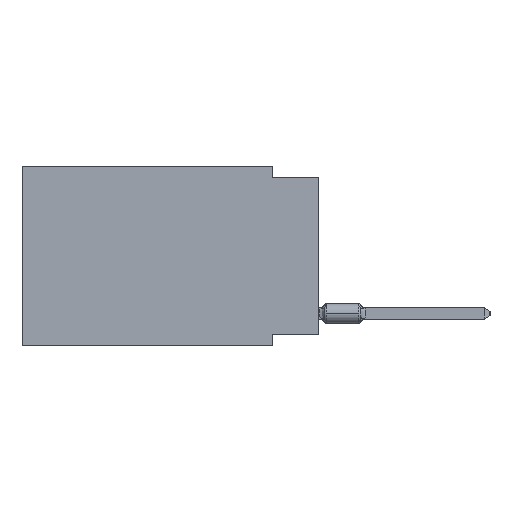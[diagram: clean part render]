
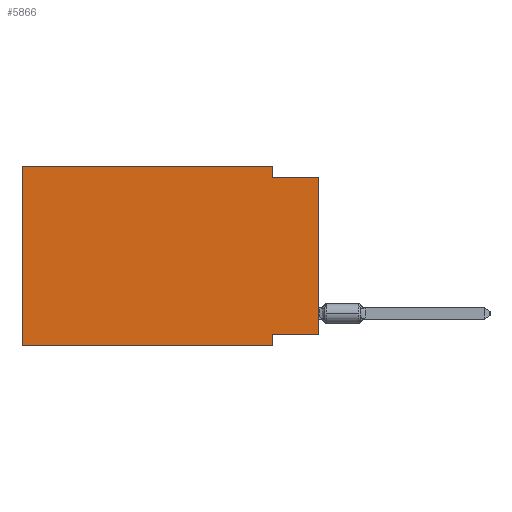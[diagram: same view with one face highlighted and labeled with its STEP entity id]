
A CAD part, left-side view. The second image highlights one B-rep face of the part: STEP entity #5866.
In plain terms, the highlighted planar face has unit normal (-1, 0, 0).
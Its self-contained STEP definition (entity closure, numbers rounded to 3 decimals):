
#885 = CARTESIAN_POINT ( 'NONE',  ( 0., 16.383, 0. ) ) ;
#1950 = CARTESIAN_POINT ( 'NONE',  ( 0., 0., -0.635 ) ) ;
#2306 = VECTOR ( 'NONE', #4783, 1000. ) ;
#2829 = EDGE_LOOP ( 'NONE', ( #25714, #37092, #14986, #3024, #22945, #7242, #21254, #27994 ) ) ;
#3024 = ORIENTED_EDGE ( 'NONE', *, *, #21896, .F. ) ;
#4580 = CARTESIAN_POINT ( 'NONE',  ( 0., 16.383, -9.906 ) ) ;
#4783 = DIRECTION ( 'NONE',  ( 0., -1., 0. ) ) ;
#4958 = DIRECTION ( 'NONE',  ( 0., 0., -1. ) ) ;
#5420 = DIRECTION ( 'NONE',  ( 0., 0., 1. ) ) ;
#5866 = ADVANCED_FACE ( 'NONE', ( #20929 ), #18463, .F. ) ;
#5921 = EDGE_CURVE ( 'NONE', #30603, #33404, #21854, .T. ) ;
#7242 = ORIENTED_EDGE ( 'NONE', *, *, #16509, .T. ) ;
#7796 = LINE ( 'NONE', #19370, #14177 ) ;
#8492 = CARTESIAN_POINT ( 'NONE',  ( 0., 2.54, -0.635 ) ) ;
#8503 = CARTESIAN_POINT ( 'NONE',  ( 0., 0., -9.271 ) ) ;
#9132 = DIRECTION ( 'NONE',  ( 0., 0., -1. ) ) ;
#9546 = CARTESIAN_POINT ( 'NONE',  ( 0., 0., -9.271 ) ) ;
#9736 = LINE ( 'NONE', #9546, #11423 ) ;
#10216 = VECTOR ( 'NONE', #9132, 1000. ) ;
#11132 = VERTEX_POINT ( 'NONE', #21292 ) ;
#11423 = VECTOR ( 'NONE', #21307, 1000. ) ;
#13697 = VECTOR ( 'NONE', #26478, 1000. ) ;
#14012 = CARTESIAN_POINT ( 'NONE',  ( 0., 0., -0.635 ) ) ;
#14177 = VECTOR ( 'NONE', #4958, 1000. ) ;
#14429 = CARTESIAN_POINT ( 'NONE',  ( 0., 2.54, -9.906 ) ) ;
#14469 = CARTESIAN_POINT ( 'NONE',  ( 0., 2.54, -9.271 ) ) ;
#14500 = EDGE_CURVE ( 'NONE', #19917, #31516, #9736, .T. ) ;
#14827 = EDGE_CURVE ( 'NONE', #33917, #30603, #23535, .T. ) ;
#14986 = ORIENTED_EDGE ( 'NONE', *, *, #14827, .F. ) ;
#16129 = CARTESIAN_POINT ( 'NONE',  ( 0., 2.54, 0. ) ) ;
#16509 = EDGE_CURVE ( 'NONE', #25045, #20562, #24486, .T. ) ;
#18463 = PLANE ( 'NONE',  #24728 ) ;
#19370 = CARTESIAN_POINT ( 'NONE',  ( 0., 2.54, -9.906 ) ) ;
#19917 = VERTEX_POINT ( 'NONE', #8503 ) ;
#20562 = VERTEX_POINT ( 'NONE', #14429 ) ;
#20722 = CARTESIAN_POINT ( 'NONE',  ( 0., 0., 0. ) ) ;
#20750 = DIRECTION ( 'NONE',  ( 0., 0., -1. ) ) ;
#20929 = FACE_OUTER_BOUND ( 'NONE', #2829, .T. ) ;
#21254 = ORIENTED_EDGE ( 'NONE', *, *, #35688, .F. ) ;
#21292 = CARTESIAN_POINT ( 'NONE',  ( 0., 16.383, 0. ) ) ;
#21307 = DIRECTION ( 'NONE',  ( 0., 1., 0. ) ) ;
#21854 = LINE ( 'NONE', #1950, #27772 ) ;
#21896 = EDGE_CURVE ( 'NONE', #11132, #33917, #23788, .T. ) ;
#22038 = DIRECTION ( 'NONE',  ( 0., -1., 0. ) ) ;
#22879 = VECTOR ( 'NONE', #5420, 1000. ) ;
#22945 = ORIENTED_EDGE ( 'NONE', *, *, #28105, .F. ) ;
#23224 = DIRECTION ( 'NONE',  ( 0., -1., 0. ) ) ;
#23535 = LINE ( 'NONE', #35084, #10216 ) ;
#23788 = LINE ( 'NONE', #32323, #24940 ) ;
#24486 = LINE ( 'NONE', #4580, #2306 ) ;
#24728 = AXIS2_PLACEMENT_3D ( 'NONE', #30013, #32485, #20750 ) ;
#24940 = VECTOR ( 'NONE', #23224, 1000. ) ;
#25045 = VERTEX_POINT ( 'NONE', #33941 ) ;
#25714 = ORIENTED_EDGE ( 'NONE', *, *, #35418, .T. ) ;
#26478 = DIRECTION ( 'NONE',  ( 0., 0., 1. ) ) ;
#27772 = VECTOR ( 'NONE', #22038, 1000. ) ;
#27994 = ORIENTED_EDGE ( 'NONE', *, *, #14500, .F. ) ;
#28105 = EDGE_CURVE ( 'NONE', #25045, #11132, #32358, .T. ) ;
#29427 = LINE ( 'NONE', #20722, #22879 ) ;
#30013 = CARTESIAN_POINT ( 'NONE',  ( 0., 16.383, 0. ) ) ;
#30603 = VERTEX_POINT ( 'NONE', #8492 ) ;
#31516 = VERTEX_POINT ( 'NONE', #14469 ) ;
#32323 = CARTESIAN_POINT ( 'NONE',  ( 0., 16.383, 0. ) ) ;
#32358 = LINE ( 'NONE', #885, #13697 ) ;
#32485 = DIRECTION ( 'NONE',  ( 1., 0., 0. ) ) ;
#33404 = VERTEX_POINT ( 'NONE', #14012 ) ;
#33917 = VERTEX_POINT ( 'NONE', #16129 ) ;
#33941 = CARTESIAN_POINT ( 'NONE',  ( 0., 16.383, -9.906 ) ) ;
#35084 = CARTESIAN_POINT ( 'NONE',  ( 0., 2.54, 0. ) ) ;
#35418 = EDGE_CURVE ( 'NONE', #19917, #33404, #29427, .T. ) ;
#35688 = EDGE_CURVE ( 'NONE', #31516, #20562, #7796, .T. ) ;
#37092 = ORIENTED_EDGE ( 'NONE', *, *, #5921, .F. ) ;
